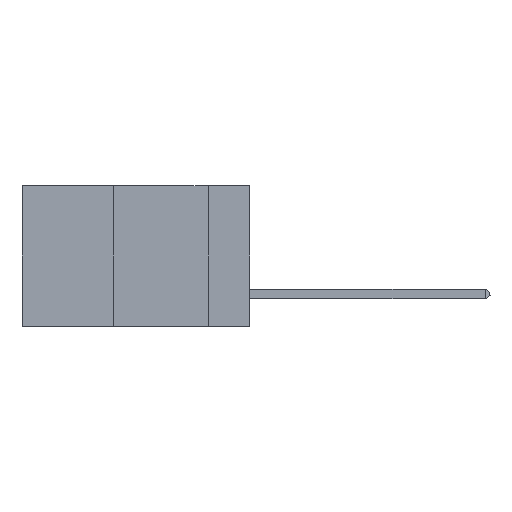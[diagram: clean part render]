
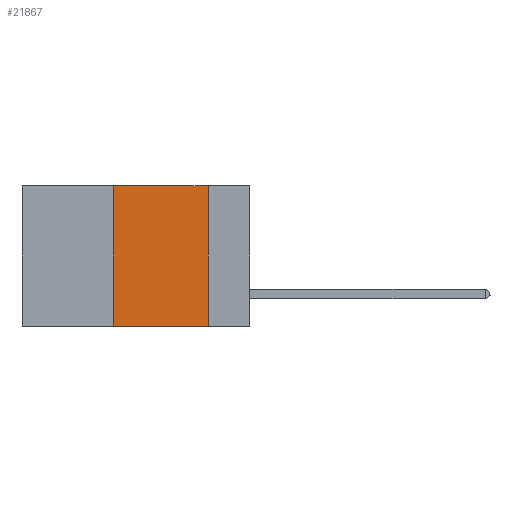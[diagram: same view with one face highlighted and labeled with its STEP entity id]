
A CAD part, left-side view. The second image highlights one B-rep face of the part: STEP entity #21867.
In plain terms, the highlighted planar face has unit normal (-1, 0, 0).
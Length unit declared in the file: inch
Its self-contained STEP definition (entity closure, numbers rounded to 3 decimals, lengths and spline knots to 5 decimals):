
#405 = CARTESIAN_POINT ( 'NONE',  ( 0., 0.36, 0. ) ) ;
#749 = LINE ( 'NONE', #1237, #6293 ) ;
#1144 = EDGE_CURVE ( 'NONE', #4794, #18926, #14147, .T. ) ;
#1237 = CARTESIAN_POINT ( 'NONE',  ( 0., 0.6, 0. ) ) ;
#1571 = PLANE ( 'NONE',  #14728 ) ;
#3134 = LINE ( 'NONE', #10103, #9972 ) ;
#4794 = VERTEX_POINT ( 'NONE', #10119 ) ;
#4832 = ORIENTED_EDGE ( 'NONE', *, *, #19173, .F. ) ;
#6293 = VECTOR ( 'NONE', #7473, 39.37008 ) ;
#7473 = DIRECTION ( 'NONE',  ( 0., -1., 0. ) ) ;
#7540 = EDGE_CURVE ( 'NONE', #4794, #8809, #3134, .T. ) ;
#7870 = EDGE_CURVE ( 'NONE', #8809, #16045, #749, .T. ) ;
#8102 = CARTESIAN_POINT ( 'NONE',  ( 0., 0.6, 0. ) ) ;
#8415 = DIRECTION ( 'NONE',  ( 0., 0., 1. ) ) ;
#8540 = CARTESIAN_POINT ( 'NONE',  ( 0., 0.11, -0.37 ) ) ;
#8745 = CARTESIAN_POINT ( 'NONE',  ( 0., 0.6, -0.37 ) ) ;
#8809 = VERTEX_POINT ( 'NONE', #405 ) ;
#8865 = VECTOR ( 'NONE', #17387, 39.37008 ) ;
#9914 = CARTESIAN_POINT ( 'NONE',  ( 0., 0.11, 0. ) ) ;
#9972 = VECTOR ( 'NONE', #8415, 39.37008 ) ;
#10103 = CARTESIAN_POINT ( 'NONE',  ( 0., 0.36, 0. ) ) ;
#10119 = CARTESIAN_POINT ( 'NONE',  ( 0., 0.36, -0.37 ) ) ;
#11356 = DIRECTION ( 'NONE',  ( 1., 0., 0. ) ) ;
#13394 = LINE ( 'NONE', #19235, #13914 ) ;
#13800 = EDGE_LOOP ( 'NONE', ( #4832, #18454, #16461, #14315 ) ) ;
#13914 = VECTOR ( 'NONE', #20966, 39.37008 ) ;
#14147 = LINE ( 'NONE', #8745, #8865 ) ;
#14315 = ORIENTED_EDGE ( 'NONE', *, *, #1144, .T. ) ;
#14728 = AXIS2_PLACEMENT_3D ( 'NONE', #8102, #11356, #19784 ) ;
#16045 = VERTEX_POINT ( 'NONE', #9914 ) ;
#16461 = ORIENTED_EDGE ( 'NONE', *, *, #7540, .F. ) ;
#17387 = DIRECTION ( 'NONE',  ( 0., -1., 0. ) ) ;
#17817 = FACE_OUTER_BOUND ( 'NONE', #13800, .T. ) ;
#18454 = ORIENTED_EDGE ( 'NONE', *, *, #7870, .F. ) ;
#18926 = VERTEX_POINT ( 'NONE', #8540 ) ;
#19173 = EDGE_CURVE ( 'NONE', #16045, #18926, #13394, .T. ) ;
#19235 = CARTESIAN_POINT ( 'NONE',  ( 0., 0.11, 0. ) ) ;
#19784 = DIRECTION ( 'NONE',  ( 0., 0., -1. ) ) ;
#20966 = DIRECTION ( 'NONE',  ( 0., 0., -1. ) ) ;
#21867 = ADVANCED_FACE ( 'NONE', ( #17817 ), #1571, .F. ) ;
